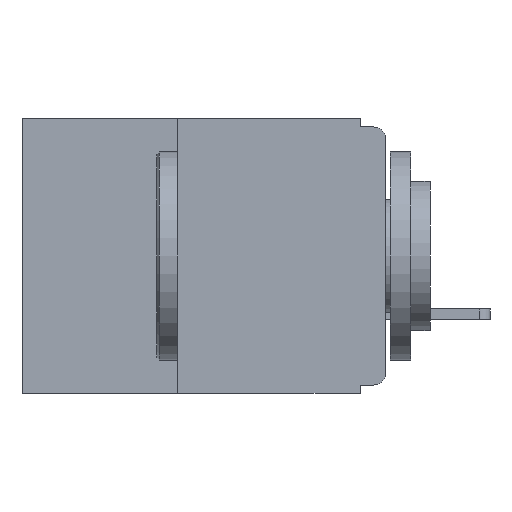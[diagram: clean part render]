
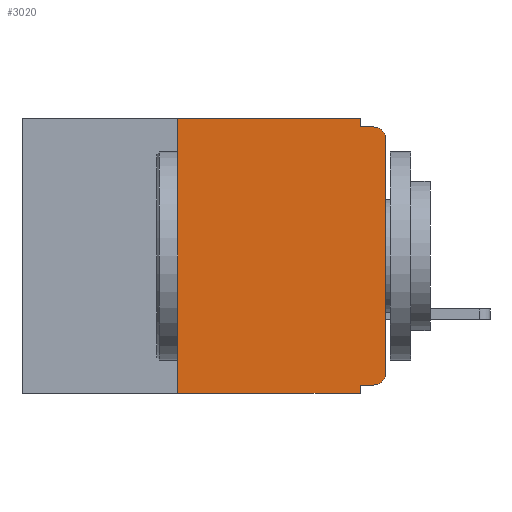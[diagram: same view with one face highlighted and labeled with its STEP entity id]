
A CAD part, left-side view. The second image highlights one B-rep face of the part: STEP entity #3020.
In plain terms, the highlighted planar face has unit normal (-1, 0, 0).
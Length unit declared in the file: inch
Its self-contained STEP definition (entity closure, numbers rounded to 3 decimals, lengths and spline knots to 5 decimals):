
#12 = EDGE_CURVE ( 'NONE', #5935, #41, #1285, .T. ) ;
#41 = VERTEX_POINT ( 'NONE', #7051 ) ;
#45 = EDGE_CURVE ( 'NONE', #3712, #1954, #1215, .T. ) ;
#69 = EDGE_CURVE ( 'NONE', #3712, #7193, #1299, .T. ) ;
#95 = EDGE_CURVE ( 'NONE', #552, #7193, #1069, .T. ) ;
#306 = LINE ( 'NONE', #9984, #12000 ) ;
#416 = DIRECTION ( 'NONE',  ( 0., 0., 1. ) ) ;
#552 = VERTEX_POINT ( 'NONE', #13397 ) ;
#639 = CARTESIAN_POINT ( 'NONE',  ( 0., 0.437, -0.33 ) ) ;
#914 = CARTESIAN_POINT ( 'NONE',  ( 0., 0.031, 0. ) ) ;
#997 = CARTESIAN_POINT ( 'NONE',  ( 0., 0., -0.32 ) ) ;
#1043 = VECTOR ( 'NONE', #13471, 39.37008 ) ;
#1069 = LINE ( 'NONE', #10247, #1043 ) ;
#1094 = VECTOR ( 'NONE', #13168, 39.37008 ) ;
#1163 = VECTOR ( 'NONE', #416, 39.37008 ) ;
#1215 = LINE ( 'NONE', #13130, #1163 ) ;
#1270 = VECTOR ( 'NONE', #12231, 39.37008 ) ;
#1285 = LINE ( 'NONE', #7700, #1270 ) ;
#1299 = LINE ( 'NONE', #639, #1094 ) ;
#1576 = LINE ( 'NONE', #997, #12790 ) ;
#1954 = VERTEX_POINT ( 'NONE', #11934 ) ;
#2233 = DIRECTION ( 'NONE',  ( -1., 0., 0. ) ) ;
#2423 = EDGE_CURVE ( 'NONE', #7237, #552, #1576, .T. ) ;
#2874 = EDGE_CURVE ( 'NONE', #1954, #5935, #9079, .T. ) ;
#3020 = ADVANCED_FACE ( 'NONE', ( #12131 ), #13858, .F. ) ;
#3220 = DIRECTION ( 'NONE',  ( 0., -1., 0. ) ) ;
#3475 = CARTESIAN_POINT ( 'NONE',  ( 0., 0.031, -0.33 ) ) ;
#3712 = VERTEX_POINT ( 'NONE', #6481 ) ;
#3726 = DIRECTION ( 'NONE',  ( 0., 0., 1. ) ) ;
#3989 = DIRECTION ( 'NONE',  ( 0., 1., 0. ) ) ;
#4391 = CIRCLE ( 'NONE', #8580, 0.015 ) ;
#4435 = CARTESIAN_POINT ( 'NONE',  ( 0., 0.437, 0. ) ) ;
#5599 = CARTESIAN_POINT ( 'NONE',  ( 0., 0., -0.305 ) ) ;
#5935 = VERTEX_POINT ( 'NONE', #914 ) ;
#5976 = CARTESIAN_POINT ( 'NONE',  ( 0., 0.437, 0. ) ) ;
#5996 = DIRECTION ( 'NONE',  ( 1., 0., 0. ) ) ;
#6349 = ORIENTED_EDGE ( 'NONE', *, *, #8042, .T. ) ;
#6374 = CARTESIAN_POINT ( 'NONE',  ( 0., 0.015, -0.305 ) ) ;
#6387 = ORIENTED_EDGE ( 'NONE', *, *, #6593, .T. ) ;
#6481 = CARTESIAN_POINT ( 'NONE',  ( 0., 0.25, -0.33 ) ) ;
#6593 = EDGE_CURVE ( 'NONE', #8517, #7440, #12132, .T. ) ;
#6637 = ORIENTED_EDGE ( 'NONE', *, *, #13741, .F. ) ;
#6681 = ORIENTED_EDGE ( 'NONE', *, *, #12, .F. ) ;
#6794 = ORIENTED_EDGE ( 'NONE', *, *, #2874, .F. ) ;
#6835 = ORIENTED_EDGE ( 'NONE', *, *, #45, .F. ) ;
#6980 = ORIENTED_EDGE ( 'NONE', *, *, #69, .T. ) ;
#7012 = ORIENTED_EDGE ( 'NONE', *, *, #95, .F. ) ;
#7040 = ORIENTED_EDGE ( 'NONE', *, *, #2423, .F. ) ;
#7051 = CARTESIAN_POINT ( 'NONE',  ( 0., 0.031, -0.01 ) ) ;
#7151 = ORIENTED_EDGE ( 'NONE', *, *, #7575, .T. ) ;
#7193 = VERTEX_POINT ( 'NONE', #3475 ) ;
#7237 = VERTEX_POINT ( 'NONE', #13847 ) ;
#7408 = VECTOR ( 'NONE', #3726, 39.37008 ) ;
#7440 = VERTEX_POINT ( 'NONE', #13249 ) ;
#7535 = DIRECTION ( 'NONE',  ( 0., 0., -1. ) ) ;
#7575 = EDGE_CURVE ( 'NONE', #7237, #7773, #4391, .T. ) ;
#7700 = CARTESIAN_POINT ( 'NONE',  ( 0., 0.031, 0. ) ) ;
#7773 = VERTEX_POINT ( 'NONE', #5599 ) ;
#8042 = EDGE_CURVE ( 'NONE', #7773, #8517, #12493, .T. ) ;
#8517 = VERTEX_POINT ( 'NONE', #8975 ) ;
#8580 = AXIS2_PLACEMENT_3D ( 'NONE', #6374, #13429, #7535 ) ;
#8975 = CARTESIAN_POINT ( 'NONE',  ( 0., 0., -0.025 ) ) ;
#9079 = LINE ( 'NONE', #4435, #13716 ) ;
#9160 = CARTESIAN_POINT ( 'NONE',  ( 0., 0.015, -0.025 ) ) ;
#9184 = DIRECTION ( 'NONE',  ( 0., 0., -1. ) ) ;
#9388 = CARTESIAN_POINT ( 'NONE',  ( 0., 0., 0. ) ) ;
#9489 = AXIS2_PLACEMENT_3D ( 'NONE', #9160, #2233, #10169 ) ;
#9984 = CARTESIAN_POINT ( 'NONE',  ( 0., 0., -0.01 ) ) ;
#10169 = DIRECTION ( 'NONE',  ( 0., 0., -1. ) ) ;
#10247 = CARTESIAN_POINT ( 'NONE',  ( 0., 0.031, -0.33 ) ) ;
#10642 = DIRECTION ( 'NONE',  ( 0., -1., 0. ) ) ;
#10760 = EDGE_LOOP ( 'NONE', ( #6349, #6387, #6637, #6681, #6794, #6835, #6980, #7012, #7040, #7151 ) ) ;
#11934 = CARTESIAN_POINT ( 'NONE',  ( 0., 0.25, 0. ) ) ;
#12000 = VECTOR ( 'NONE', #3220, 39.37008 ) ;
#12131 = FACE_OUTER_BOUND ( 'NONE', #10760, .T. ) ;
#12132 = CIRCLE ( 'NONE', #9489, 0.015 ) ;
#12231 = DIRECTION ( 'NONE',  ( 0., 0., -1. ) ) ;
#12493 = LINE ( 'NONE', #9388, #7408 ) ;
#12790 = VECTOR ( 'NONE', #3989, 39.37008 ) ;
#13130 = CARTESIAN_POINT ( 'NONE',  ( 0., 0.25, -0.33 ) ) ;
#13168 = DIRECTION ( 'NONE',  ( 0., -1., 0. ) ) ;
#13249 = CARTESIAN_POINT ( 'NONE',  ( 0., 0.015, -0.01 ) ) ;
#13397 = CARTESIAN_POINT ( 'NONE',  ( 0., 0.031, -0.32 ) ) ;
#13429 = DIRECTION ( 'NONE',  ( -1., 0., 0. ) ) ;
#13471 = DIRECTION ( 'NONE',  ( 0., 0., -1. ) ) ;
#13630 = AXIS2_PLACEMENT_3D ( 'NONE', #5976, #5996, #9184 ) ;
#13716 = VECTOR ( 'NONE', #10642, 39.37008 ) ;
#13741 = EDGE_CURVE ( 'NONE', #41, #7440, #306, .T. ) ;
#13847 = CARTESIAN_POINT ( 'NONE',  ( 0., 0.015, -0.32 ) ) ;
#13858 = PLANE ( 'NONE',  #13630 ) ;
